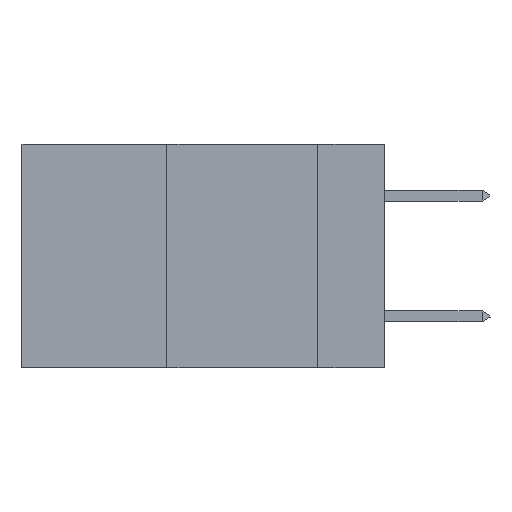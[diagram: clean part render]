
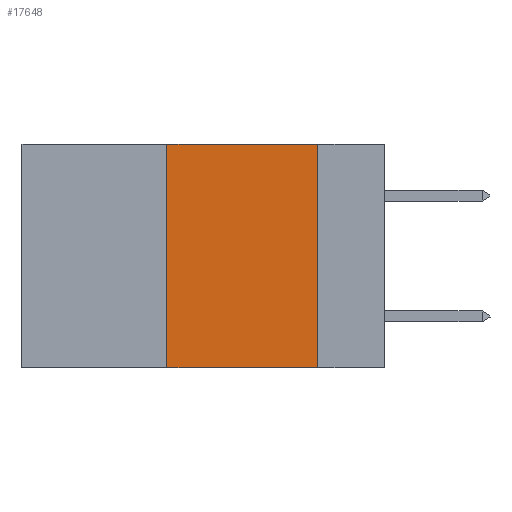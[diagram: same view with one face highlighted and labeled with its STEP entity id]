
A CAD part, left-side view. The second image highlights one B-rep face of the part: STEP entity #17648.
In plain terms, the highlighted planar face has unit normal (-1, 0, 0).
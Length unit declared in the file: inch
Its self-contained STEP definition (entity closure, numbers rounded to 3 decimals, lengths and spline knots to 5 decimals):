
#150 = FACE_OUTER_BOUND ( 'NONE', #15532, .T. ) ;
#1614 = LINE ( 'NONE', #21845, #6268 ) ;
#1630 = ORIENTED_EDGE ( 'NONE', *, *, #16474, .F. ) ;
#2631 = DIRECTION ( 'NONE',  ( 0., -1., 0. ) ) ;
#3286 = DIRECTION ( 'NONE',  ( 1., 0., 0. ) ) ;
#3644 = DIRECTION ( 'NONE',  ( 0., -1., 0. ) ) ;
#4507 = VECTOR ( 'NONE', #13758, 39.37008 ) ;
#5152 = VECTOR ( 'NONE', #3644, 39.37008 ) ;
#6268 = VECTOR ( 'NONE', #11848, 39.37008 ) ;
#6281 = ORIENTED_EDGE ( 'NONE', *, *, #7057, .T. ) ;
#7057 = EDGE_CURVE ( 'NONE', #15522, #9269, #11300, .T. ) ;
#7126 = CARTESIAN_POINT ( 'NONE',  ( 0., 0.6, 0. ) ) ;
#8512 = LINE ( 'NONE', #12112, #4507 ) ;
#9269 = VERTEX_POINT ( 'NONE', #11738 ) ;
#9479 = EDGE_CURVE ( 'NONE', #19767, #18681, #9677, .T. ) ;
#9677 = LINE ( 'NONE', #7126, #5152 ) ;
#9737 = ORIENTED_EDGE ( 'NONE', *, *, #11279, .F. ) ;
#10156 = PLANE ( 'NONE',  #19926 ) ;
#11279 = EDGE_CURVE ( 'NONE', #18681, #9269, #8512, .T. ) ;
#11300 = LINE ( 'NONE', #17927, #20169 ) ;
#11738 = CARTESIAN_POINT ( 'NONE',  ( 0., 0.11, -0.37 ) ) ;
#11821 = CARTESIAN_POINT ( 'NONE',  ( 0., 0.6, 0. ) ) ;
#11848 = DIRECTION ( 'NONE',  ( 0., 0., 1. ) ) ;
#12112 = CARTESIAN_POINT ( 'NONE',  ( 0., 0.11, 0. ) ) ;
#13758 = DIRECTION ( 'NONE',  ( 0., 0., -1. ) ) ;
#15147 = DIRECTION ( 'NONE',  ( 0., 0., -1. ) ) ;
#15522 = VERTEX_POINT ( 'NONE', #19504 ) ;
#15532 = EDGE_LOOP ( 'NONE', ( #9737, #18652, #1630, #6281 ) ) ;
#16161 = CARTESIAN_POINT ( 'NONE',  ( 0., 0.36, 0. ) ) ;
#16474 = EDGE_CURVE ( 'NONE', #15522, #19767, #1614, .T. ) ;
#17648 = ADVANCED_FACE ( 'NONE', ( #150 ), #10156, .F. ) ;
#17927 = CARTESIAN_POINT ( 'NONE',  ( 0., 0.6, -0.37 ) ) ;
#18652 = ORIENTED_EDGE ( 'NONE', *, *, #9479, .F. ) ;
#18681 = VERTEX_POINT ( 'NONE', #21358 ) ;
#19504 = CARTESIAN_POINT ( 'NONE',  ( 0., 0.36, -0.37 ) ) ;
#19767 = VERTEX_POINT ( 'NONE', #16161 ) ;
#19926 = AXIS2_PLACEMENT_3D ( 'NONE', #11821, #3286, #15147 ) ;
#20169 = VECTOR ( 'NONE', #2631, 39.37008 ) ;
#21358 = CARTESIAN_POINT ( 'NONE',  ( 0., 0.11, 0. ) ) ;
#21845 = CARTESIAN_POINT ( 'NONE',  ( 0., 0.36, 0. ) ) ;
